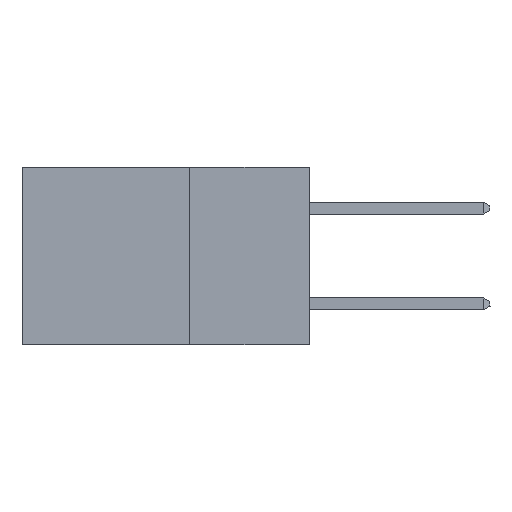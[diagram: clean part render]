
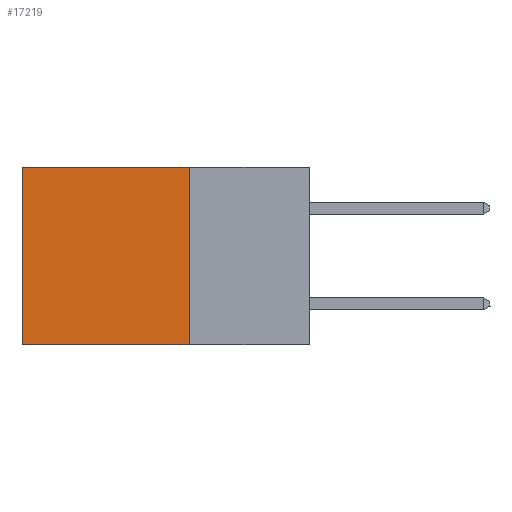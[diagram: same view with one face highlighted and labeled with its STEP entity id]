
A CAD part, left-side view. The second image highlights one B-rep face of the part: STEP entity #17219.
In plain terms, the highlighted planar face has unit normal (-1, 0, 0).
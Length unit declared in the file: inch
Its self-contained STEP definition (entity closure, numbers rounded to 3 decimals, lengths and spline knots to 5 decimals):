
#114 = EDGE_CURVE ( 'NONE', #25046, #10530, #20463, .T. ) ;
#1145 = ORIENTED_EDGE ( 'NONE', *, *, #15944, .F. ) ;
#1942 = CARTESIAN_POINT ( 'NONE',  ( 0.2875, 0.6, -0.37 ) ) ;
#1949 = PLANE ( 'NONE',  #8995 ) ;
#2012 = VECTOR ( 'NONE', #12728, 39.37008 ) ;
#2032 = DIRECTION ( 'NONE',  ( 1., 0., 0. ) ) ;
#3299 = CARTESIAN_POINT ( 'NONE',  ( 0.2875, 0.25, 0. ) ) ;
#3747 = VECTOR ( 'NONE', #21264, 39.37008 ) ;
#3870 = EDGE_LOOP ( 'NONE', ( #25160, #1145, #11342, #22023 ) ) ;
#5320 = CARTESIAN_POINT ( 'NONE',  ( 0.2875, 0.25, -0.37 ) ) ;
#6336 = DIRECTION ( 'NONE',  ( 0., 1., 0. ) ) ;
#6796 = EDGE_CURVE ( 'NONE', #25046, #11551, #16593, .T. ) ;
#8154 = LINE ( 'NONE', #14838, #13397 ) ;
#8652 = FACE_OUTER_BOUND ( 'NONE', #3870, .T. ) ;
#8995 = AXIS2_PLACEMENT_3D ( 'NONE', #25061, #2032, #10120 ) ;
#10120 = DIRECTION ( 'NONE',  ( 0., 0., -1. ) ) ;
#10530 = VERTEX_POINT ( 'NONE', #5320 ) ;
#11342 = ORIENTED_EDGE ( 'NONE', *, *, #114, .F. ) ;
#11551 = VERTEX_POINT ( 'NONE', #15535 ) ;
#11989 = EDGE_CURVE ( 'NONE', #11551, #23679, #20240, .T. ) ;
#12476 = CARTESIAN_POINT ( 'NONE',  ( 0.2875, 0.6, 0. ) ) ;
#12728 = DIRECTION ( 'NONE',  ( 0., 0., -1. ) ) ;
#13397 = VECTOR ( 'NONE', #6336, 39.37008 ) ;
#13668 = VECTOR ( 'NONE', #26038, 39.37008 ) ;
#14838 = CARTESIAN_POINT ( 'NONE',  ( 0.2875, 0.25, -0.37 ) ) ;
#15535 = CARTESIAN_POINT ( 'NONE',  ( 0.2875, 0.6, 0. ) ) ;
#15944 = EDGE_CURVE ( 'NONE', #10530, #23679, #8154, .T. ) ;
#16593 = LINE ( 'NONE', #3299, #13668 ) ;
#17219 = ADVANCED_FACE ( 'NONE', ( #8652 ), #1949, .F. ) ;
#18894 = CARTESIAN_POINT ( 'NONE',  ( 0.2875, 0.25, 0. ) ) ;
#20240 = LINE ( 'NONE', #12476, #3747 ) ;
#20463 = LINE ( 'NONE', #25239, #2012 ) ;
#21264 = DIRECTION ( 'NONE',  ( 0., 0., -1. ) ) ;
#22023 = ORIENTED_EDGE ( 'NONE', *, *, #6796, .T. ) ;
#23679 = VERTEX_POINT ( 'NONE', #1942 ) ;
#25046 = VERTEX_POINT ( 'NONE', #18894 ) ;
#25061 = CARTESIAN_POINT ( 'NONE',  ( 0.2875, 0.25, 0. ) ) ;
#25160 = ORIENTED_EDGE ( 'NONE', *, *, #11989, .T. ) ;
#25239 = CARTESIAN_POINT ( 'NONE',  ( 0.2875, 0.25, 0. ) ) ;
#26038 = DIRECTION ( 'NONE',  ( 0., 1., 0. ) ) ;
